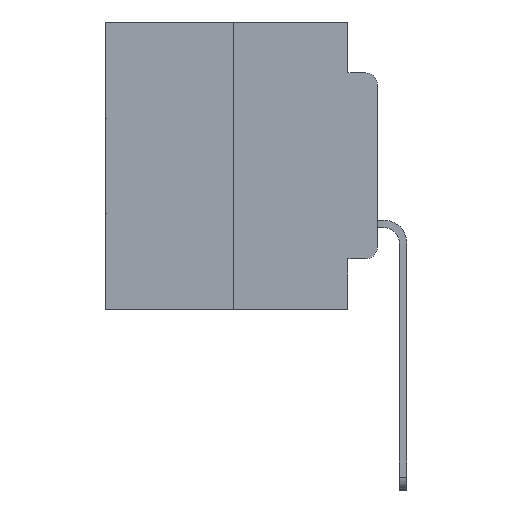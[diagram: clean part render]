
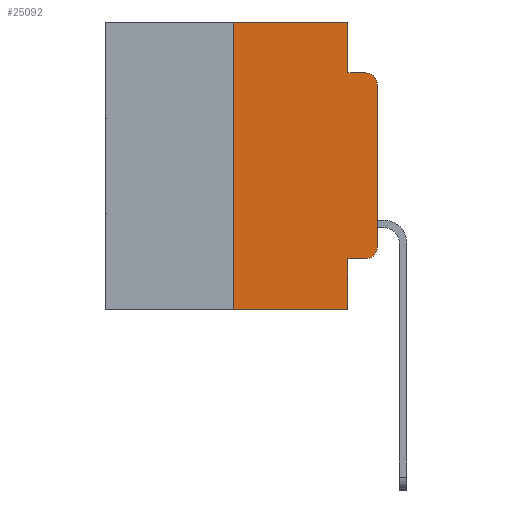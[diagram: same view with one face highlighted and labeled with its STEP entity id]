
A CAD part, left-side view. The second image highlights one B-rep face of the part: STEP entity #25092.
In plain terms, the highlighted planar face has unit normal (-1, 0, 0).
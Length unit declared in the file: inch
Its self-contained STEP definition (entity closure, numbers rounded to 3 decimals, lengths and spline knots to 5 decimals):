
#196 = LINE ( 'NONE', #7297, #18007 ) ;
#404 = VECTOR ( 'NONE', #4435, 39.37008 ) ;
#434 = CARTESIAN_POINT ( 'NONE',  ( 0., 0.051, -0.4115 ) ) ;
#594 = PLANE ( 'NONE',  #27702 ) ;
#703 = DIRECTION ( 'NONE',  ( 1., 0., 0. ) ) ;
#1076 = DIRECTION ( 'NONE',  ( 0., 0., -1. ) ) ;
#1322 = VERTEX_POINT ( 'NONE', #434 ) ;
#1398 = CARTESIAN_POINT ( 'NONE',  ( 0., 0.051, 0. ) ) ;
#1794 = LINE ( 'NONE', #1398, #25560 ) ;
#1905 = VECTOR ( 'NONE', #11629, 39.37008 ) ;
#2314 = EDGE_CURVE ( 'NONE', #7797, #24586, #27028, .T. ) ;
#2492 = AXIS2_PLACEMENT_3D ( 'NONE', #26879, #13303, #29120 ) ;
#2726 = ORIENTED_EDGE ( 'NONE', *, *, #10645, .T. ) ;
#2782 = EDGE_CURVE ( 'NONE', #1322, #9401, #1794, .T. ) ;
#2810 = VERTEX_POINT ( 'NONE', #19928 ) ;
#2855 = LINE ( 'NONE', #23518, #21236 ) ;
#3031 = LINE ( 'NONE', #6026, #14648 ) ;
#3638 = DIRECTION ( 'NONE',  ( 0., -1., 0. ) ) ;
#3828 = DIRECTION ( 'NONE',  ( 0., 0., -1. ) ) ;
#4218 = ORIENTED_EDGE ( 'NONE', *, *, #18549, .T. ) ;
#4435 = DIRECTION ( 'NONE',  ( 0., 0., 1. ) ) ;
#4637 = LINE ( 'NONE', #6196, #28207 ) ;
#4736 = ORIENTED_EDGE ( 'NONE', *, *, #2782, .F. ) ;
#4876 = VERTEX_POINT ( 'NONE', #26349 ) ;
#4975 = EDGE_CURVE ( 'NONE', #2810, #13143, #4637, .T. ) ;
#5012 = CARTESIAN_POINT ( 'NONE',  ( 0., 0.02, -0.0885 ) ) ;
#6026 = CARTESIAN_POINT ( 'NONE',  ( 0., 0.051, -0.0885 ) ) ;
#6196 = CARTESIAN_POINT ( 'NONE',  ( 0., 0.25, 0. ) ) ;
#7297 = CARTESIAN_POINT ( 'NONE',  ( 0., 0.473, -0.5 ) ) ;
#7311 = ORIENTED_EDGE ( 'NONE', *, *, #13422, .T. ) ;
#7797 = VERTEX_POINT ( 'NONE', #19029 ) ;
#8349 = ORIENTED_EDGE ( 'NONE', *, *, #27703, .F. ) ;
#8501 = ORIENTED_EDGE ( 'NONE', *, *, #9458, .F. ) ;
#9401 = VERTEX_POINT ( 'NONE', #25018 ) ;
#9458 = EDGE_CURVE ( 'NONE', #4876, #17199, #28461, .T. ) ;
#9496 = CARTESIAN_POINT ( 'NONE',  ( 0., 0.051, -0.4115 ) ) ;
#9767 = VECTOR ( 'NONE', #13979, 39.37008 ) ;
#10645 = EDGE_CURVE ( 'NONE', #12668, #16697, #22388, .T. ) ;
#11629 = DIRECTION ( 'NONE',  ( 0., 0., -1. ) ) ;
#12668 = VERTEX_POINT ( 'NONE', #25144 ) ;
#13143 = VERTEX_POINT ( 'NONE', #22128 ) ;
#13303 = DIRECTION ( 'NONE',  ( -1., 0., 0. ) ) ;
#13422 = EDGE_CURVE ( 'NONE', #1322, #7797, #28551, .T. ) ;
#13488 = AXIS2_PLACEMENT_3D ( 'NONE', #28606, #15050, #1076 ) ;
#13896 = CARTESIAN_POINT ( 'NONE',  ( 0., 0.051, 0. ) ) ;
#13979 = DIRECTION ( 'NONE',  ( 0., -1., 0. ) ) ;
#14648 = VECTOR ( 'NONE', #3638, 39.37008 ) ;
#15050 = DIRECTION ( 'NONE',  ( -1., 0., 0. ) ) ;
#15088 = ORIENTED_EDGE ( 'NONE', *, *, #24329, .T. ) ;
#15214 = CARTESIAN_POINT ( 'NONE',  ( 0., 0., -0.3915 ) ) ;
#15266 = EDGE_CURVE ( 'NONE', #13143, #4876, #2855, .T. ) ;
#15887 = FACE_OUTER_BOUND ( 'NONE', #26612, .T. ) ;
#16697 = VERTEX_POINT ( 'NONE', #5012 ) ;
#16969 = DIRECTION ( 'NONE',  ( 0., 0., -1. ) ) ;
#17199 = VERTEX_POINT ( 'NONE', #27645 ) ;
#18007 = VECTOR ( 'NONE', #25648, 39.37008 ) ;
#18184 = CARTESIAN_POINT ( 'NONE',  ( 0., 0., 0. ) ) ;
#18549 = EDGE_CURVE ( 'NONE', #24586, #12668, #24272, .T. ) ;
#19029 = CARTESIAN_POINT ( 'NONE',  ( 0., 0.02, -0.4115 ) ) ;
#19160 = CARTESIAN_POINT ( 'NONE',  ( 0., 0.473, 0. ) ) ;
#19928 = CARTESIAN_POINT ( 'NONE',  ( 0., 0.25, -0.5 ) ) ;
#21236 = VECTOR ( 'NONE', #28033, 39.37008 ) ;
#22128 = CARTESIAN_POINT ( 'NONE',  ( 0., 0.25, 0. ) ) ;
#22388 = CIRCLE ( 'NONE', #13488, 0.02 ) ;
#23518 = CARTESIAN_POINT ( 'NONE',  ( 0., 0.473, 0. ) ) ;
#24243 = ORIENTED_EDGE ( 'NONE', *, *, #4975, .F. ) ;
#24272 = LINE ( 'NONE', #18184, #404 ) ;
#24329 = EDGE_CURVE ( 'NONE', #2810, #9401, #196, .T. ) ;
#24486 = DIRECTION ( 'NONE',  ( 0., 0., 1. ) ) ;
#24586 = VERTEX_POINT ( 'NONE', #15214 ) ;
#25018 = CARTESIAN_POINT ( 'NONE',  ( 0., 0.051, -0.5 ) ) ;
#25092 = ADVANCED_FACE ( 'NONE', ( #15887 ), #594, .F. ) ;
#25144 = CARTESIAN_POINT ( 'NONE',  ( 0., 0., -0.1085 ) ) ;
#25431 = ORIENTED_EDGE ( 'NONE', *, *, #2314, .T. ) ;
#25560 = VECTOR ( 'NONE', #3828, 39.37008 ) ;
#25648 = DIRECTION ( 'NONE',  ( 0., -1., 0. ) ) ;
#26349 = CARTESIAN_POINT ( 'NONE',  ( 0., 0.051, 0. ) ) ;
#26612 = EDGE_LOOP ( 'NONE', ( #4218, #2726, #8349, #8501, #28521, #24243, #15088, #4736, #7311, #25431 ) ) ;
#26879 = CARTESIAN_POINT ( 'NONE',  ( 0., 0.02, -0.3915 ) ) ;
#27028 = CIRCLE ( 'NONE', #2492, 0.02 ) ;
#27645 = CARTESIAN_POINT ( 'NONE',  ( 0., 0.051, -0.0885 ) ) ;
#27702 = AXIS2_PLACEMENT_3D ( 'NONE', #19160, #703, #16969 ) ;
#27703 = EDGE_CURVE ( 'NONE', #17199, #16697, #3031, .T. ) ;
#28033 = DIRECTION ( 'NONE',  ( 0., -1., 0. ) ) ;
#28207 = VECTOR ( 'NONE', #24486, 39.37008 ) ;
#28461 = LINE ( 'NONE', #13896, #1905 ) ;
#28521 = ORIENTED_EDGE ( 'NONE', *, *, #15266, .F. ) ;
#28551 = LINE ( 'NONE', #9496, #9767 ) ;
#28606 = CARTESIAN_POINT ( 'NONE',  ( 0., 0.02, -0.1085 ) ) ;
#29120 = DIRECTION ( 'NONE',  ( 0., 0., -1. ) ) ;
